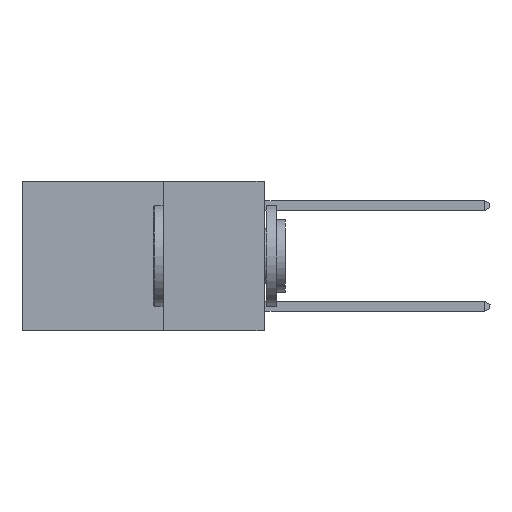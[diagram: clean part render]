
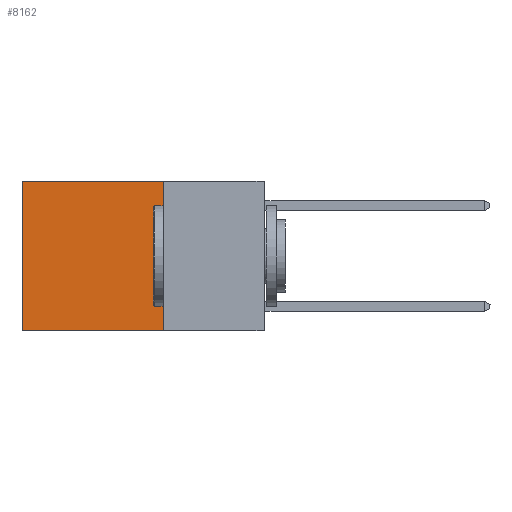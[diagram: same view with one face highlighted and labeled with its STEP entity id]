
A CAD part, left-side view. The second image highlights one B-rep face of the part: STEP entity #8162.
In plain terms, the highlighted planar face has unit normal (-1, 0, 0).
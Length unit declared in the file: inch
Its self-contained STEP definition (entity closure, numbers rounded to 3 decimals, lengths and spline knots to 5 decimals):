
#136 = ORIENTED_EDGE ( 'NONE', *, *, #281, .F. ) ;
#160 = VERTEX_POINT ( 'NONE', #4352 ) ;
#281 = EDGE_CURVE ( 'NONE', #614, #5250, #2379, .T. ) ;
#614 = VERTEX_POINT ( 'NONE', #10871 ) ;
#1376 = DIRECTION ( 'NONE',  ( 0., 0., -1. ) ) ;
#1496 = LINE ( 'NONE', #2894, #11544 ) ;
#2176 = VERTEX_POINT ( 'NONE', #12138 ) ;
#2313 = CARTESIAN_POINT ( 'NONE',  ( 0.2625, 0.25, -0.37 ) ) ;
#2379 = LINE ( 'NONE', #2313, #10000 ) ;
#2894 = CARTESIAN_POINT ( 'NONE',  ( 0.2625, 0.25, 0. ) ) ;
#3124 = LINE ( 'NONE', #5150, #10465 ) ;
#3378 = DIRECTION ( 'NONE',  ( 0., 0., -1. ) ) ;
#4348 = ORIENTED_EDGE ( 'NONE', *, *, #11482, .T. ) ;
#4352 = CARTESIAN_POINT ( 'NONE',  ( 0.2625, 0.6, 0. ) ) ;
#4770 = ORIENTED_EDGE ( 'NONE', *, *, #10559, .F. ) ;
#5150 = CARTESIAN_POINT ( 'NONE',  ( 0.2625, 0.25, 0. ) ) ;
#5250 = VERTEX_POINT ( 'NONE', #10045 ) ;
#5295 = EDGE_LOOP ( 'NONE', ( #4348, #136, #4770, #9152 ) ) ;
#6178 = DIRECTION ( 'NONE',  ( 0., 0., -1. ) ) ;
#6392 = CARTESIAN_POINT ( 'NONE',  ( 0.2625, 0.6, 0. ) ) ;
#6940 = DIRECTION ( 'NONE',  ( 0., 1., 0. ) ) ;
#7429 = DIRECTION ( 'NONE',  ( 1., 0., 0. ) ) ;
#7800 = VECTOR ( 'NONE', #3378, 39.37008 ) ;
#8162 = ADVANCED_FACE ( 'NONE', ( #12518 ), #11375, .F. ) ;
#9111 = EDGE_CURVE ( 'NONE', #2176, #160, #1496, .T. ) ;
#9152 = ORIENTED_EDGE ( 'NONE', *, *, #9111, .T. ) ;
#9835 = DIRECTION ( 'NONE',  ( 0., 1., 0. ) ) ;
#10000 = VECTOR ( 'NONE', #6940, 39.37008 ) ;
#10045 = CARTESIAN_POINT ( 'NONE',  ( 0.2625, 0.6, -0.37 ) ) ;
#10440 = LINE ( 'NONE', #6392, #7800 ) ;
#10465 = VECTOR ( 'NONE', #6178, 39.37008 ) ;
#10559 = EDGE_CURVE ( 'NONE', #2176, #614, #3124, .T. ) ;
#10871 = CARTESIAN_POINT ( 'NONE',  ( 0.2625, 0.25, -0.37 ) ) ;
#10993 = AXIS2_PLACEMENT_3D ( 'NONE', #12400, #7429, #1376 ) ;
#11375 = PLANE ( 'NONE',  #10993 ) ;
#11482 = EDGE_CURVE ( 'NONE', #160, #5250, #10440, .T. ) ;
#11544 = VECTOR ( 'NONE', #9835, 39.37008 ) ;
#12138 = CARTESIAN_POINT ( 'NONE',  ( 0.2625, 0.25, 0. ) ) ;
#12400 = CARTESIAN_POINT ( 'NONE',  ( 0.2625, 0.25, 0. ) ) ;
#12518 = FACE_OUTER_BOUND ( 'NONE', #5295, .T. ) ;
